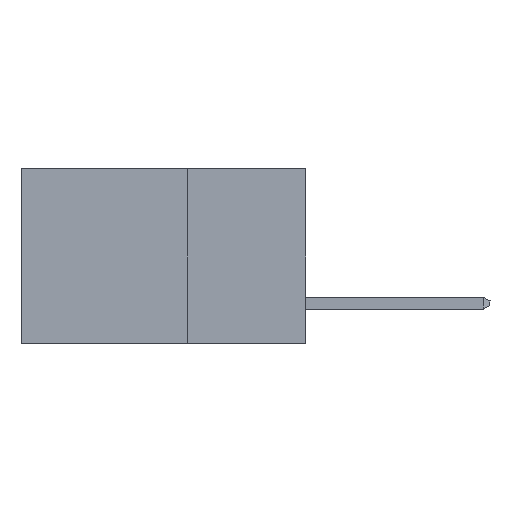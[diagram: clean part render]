
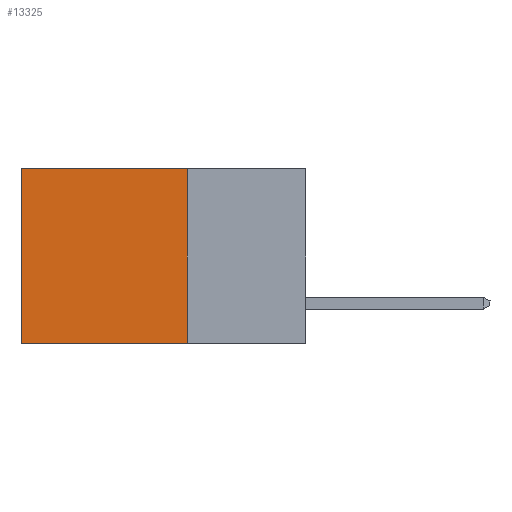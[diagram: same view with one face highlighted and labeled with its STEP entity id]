
A CAD part, left-side view. The second image highlights one B-rep face of the part: STEP entity #13325.
In plain terms, the highlighted planar face has unit normal (-1, 0, 0).
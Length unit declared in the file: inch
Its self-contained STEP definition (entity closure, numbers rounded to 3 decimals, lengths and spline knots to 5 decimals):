
#202 = EDGE_CURVE ( 'NONE', #18273, #12351, #2271, .T. ) ;
#693 = VECTOR ( 'NONE', #1187, 39.37008 ) ;
#1187 = DIRECTION ( 'NONE',  ( 0., 1., 0. ) ) ;
#1848 = VERTEX_POINT ( 'NONE', #16725 ) ;
#2271 = LINE ( 'NONE', #8118, #3606 ) ;
#3187 = FACE_OUTER_BOUND ( 'NONE', #9073, .T. ) ;
#3590 = VECTOR ( 'NONE', #4410, 39.37008 ) ;
#3606 = VECTOR ( 'NONE', #15718, 39.37008 ) ;
#3767 = ORIENTED_EDGE ( 'NONE', *, *, #202, .F. ) ;
#4410 = DIRECTION ( 'NONE',  ( 0., 1., 0. ) ) ;
#5743 = CARTESIAN_POINT ( 'NONE',  ( 0.2615, 0.25, -0.37 ) ) ;
#6311 = VERTEX_POINT ( 'NONE', #7877 ) ;
#6323 = DIRECTION ( 'NONE',  ( 1., 0., 0. ) ) ;
#6826 = CARTESIAN_POINT ( 'NONE',  ( 0.2615, 0.25, -0.37 ) ) ;
#7877 = CARTESIAN_POINT ( 'NONE',  ( 0.2615, 0.6, -0.37 ) ) ;
#8118 = CARTESIAN_POINT ( 'NONE',  ( 0.2615, 0.25, -0.37 ) ) ;
#9073 = EDGE_LOOP ( 'NONE', ( #17266, #17358, #3767, #15515 ) ) ;
#9107 = PLANE ( 'NONE',  #18639 ) ;
#9443 = LINE ( 'NONE', #10781, #13446 ) ;
#9937 = EDGE_CURVE ( 'NONE', #18273, #1848, #11354, .T. ) ;
#10619 = CARTESIAN_POINT ( 'NONE',  ( 0.2615, 0.25, -0.37 ) ) ;
#10781 = CARTESIAN_POINT ( 'NONE',  ( 0.2615, 0.6, -0.37 ) ) ;
#11354 = LINE ( 'NONE', #17418, #693 ) ;
#11545 = EDGE_CURVE ( 'NONE', #12351, #6311, #11570, .T. ) ;
#11570 = LINE ( 'NONE', #5743, #3590 ) ;
#12351 = VERTEX_POINT ( 'NONE', #6826 ) ;
#12773 = CARTESIAN_POINT ( 'NONE',  ( 0.2615, 0.25, 0. ) ) ;
#13325 = ADVANCED_FACE ( 'NONE', ( #3187 ), #9107, .F. ) ;
#13446 = VECTOR ( 'NONE', #15214, 39.37008 ) ;
#15214 = DIRECTION ( 'NONE',  ( 0., 0., -1. ) ) ;
#15515 = ORIENTED_EDGE ( 'NONE', *, *, #9937, .T. ) ;
#15718 = DIRECTION ( 'NONE',  ( 0., 0., -1. ) ) ;
#16397 = EDGE_CURVE ( 'NONE', #1848, #6311, #9443, .T. ) ;
#16725 = CARTESIAN_POINT ( 'NONE',  ( 0.2615, 0.6, 0. ) ) ;
#17266 = ORIENTED_EDGE ( 'NONE', *, *, #16397, .T. ) ;
#17358 = ORIENTED_EDGE ( 'NONE', *, *, #11545, .F. ) ;
#17418 = CARTESIAN_POINT ( 'NONE',  ( 0.2615, 0.25, 0. ) ) ;
#18019 = DIRECTION ( 'NONE',  ( 0., 0., -1. ) ) ;
#18273 = VERTEX_POINT ( 'NONE', #12773 ) ;
#18639 = AXIS2_PLACEMENT_3D ( 'NONE', #10619, #6323, #18019 ) ;
